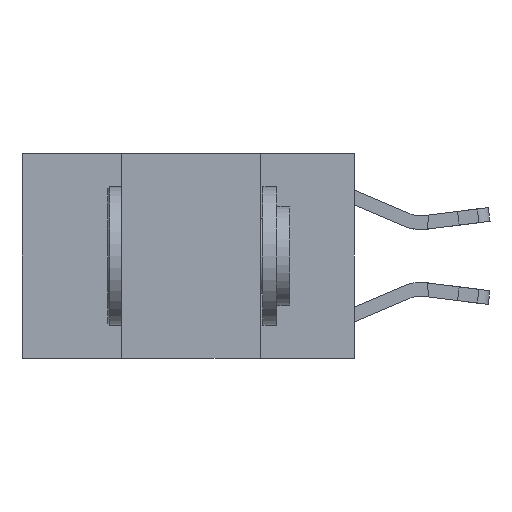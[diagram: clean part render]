
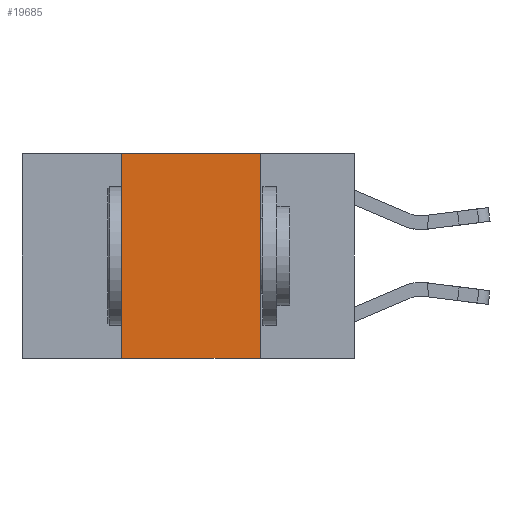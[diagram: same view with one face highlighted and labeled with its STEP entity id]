
A CAD part, left-side view. The second image highlights one B-rep face of the part: STEP entity #19685.
In plain terms, the highlighted planar face has unit normal (-1, 0, 0).
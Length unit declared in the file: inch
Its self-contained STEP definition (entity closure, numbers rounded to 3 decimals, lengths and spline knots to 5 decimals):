
#281 = CARTESIAN_POINT ( 'NONE',  ( 0., 0.6, -0.37 ) ) ;
#896 = CARTESIAN_POINT ( 'NONE',  ( 0., 0.17, -0.37 ) ) ;
#1471 = CARTESIAN_POINT ( 'NONE',  ( 0., 0.42, 0. ) ) ;
#1798 = VERTEX_POINT ( 'NONE', #6641 ) ;
#2816 = DIRECTION ( 'NONE',  ( 0., 0., -1. ) ) ;
#3092 = LINE ( 'NONE', #1471, #21780 ) ;
#3504 = AXIS2_PLACEMENT_3D ( 'NONE', #6647, #8461, #21162 ) ;
#4571 = ORIENTED_EDGE ( 'NONE', *, *, #18219, .F. ) ;
#4641 = CARTESIAN_POINT ( 'NONE',  ( 0., 0.17, 0. ) ) ;
#4829 = PLANE ( 'NONE',  #3504 ) ;
#5236 = EDGE_CURVE ( 'NONE', #16863, #1798, #23052, .T. ) ;
#5339 = CARTESIAN_POINT ( 'NONE',  ( 0., 0.6, 0. ) ) ;
#6197 = LINE ( 'NONE', #4641, #15296 ) ;
#6641 = CARTESIAN_POINT ( 'NONE',  ( 0., 0.17, 0. ) ) ;
#6647 = CARTESIAN_POINT ( 'NONE',  ( 0., 0.6, 0. ) ) ;
#7372 = VERTEX_POINT ( 'NONE', #896 ) ;
#8461 = DIRECTION ( 'NONE',  ( 1., 0., 0. ) ) ;
#8609 = EDGE_CURVE ( 'NONE', #1798, #7372, #6197, .T. ) ;
#9199 = VECTOR ( 'NONE', #12646, 39.37008 ) ;
#10475 = DIRECTION ( 'NONE',  ( 0., 0., 1. ) ) ;
#11196 = DIRECTION ( 'NONE',  ( 0., -1., 0. ) ) ;
#12395 = ORIENTED_EDGE ( 'NONE', *, *, #8609, .F. ) ;
#12646 = DIRECTION ( 'NONE',  ( 0., -1., 0. ) ) ;
#12648 = VERTEX_POINT ( 'NONE', #18712 ) ;
#13178 = LINE ( 'NONE', #281, #18047 ) ;
#15296 = VECTOR ( 'NONE', #2816, 39.37008 ) ;
#15755 = EDGE_CURVE ( 'NONE', #12648, #7372, #13178, .T. ) ;
#16863 = VERTEX_POINT ( 'NONE', #23302 ) ;
#18047 = VECTOR ( 'NONE', #11196, 39.37008 ) ;
#18123 = EDGE_LOOP ( 'NONE', ( #12395, #19794, #4571, #21141 ) ) ;
#18219 = EDGE_CURVE ( 'NONE', #12648, #16863, #3092, .T. ) ;
#18712 = CARTESIAN_POINT ( 'NONE',  ( 0., 0.42, -0.37 ) ) ;
#19685 = ADVANCED_FACE ( 'NONE', ( #20614 ), #4829, .F. ) ;
#19794 = ORIENTED_EDGE ( 'NONE', *, *, #5236, .F. ) ;
#20614 = FACE_OUTER_BOUND ( 'NONE', #18123, .T. ) ;
#21141 = ORIENTED_EDGE ( 'NONE', *, *, #15755, .T. ) ;
#21162 = DIRECTION ( 'NONE',  ( 0., 0., -1. ) ) ;
#21780 = VECTOR ( 'NONE', #10475, 39.37008 ) ;
#23052 = LINE ( 'NONE', #5339, #9199 ) ;
#23302 = CARTESIAN_POINT ( 'NONE',  ( 0., 0.42, 0. ) ) ;
